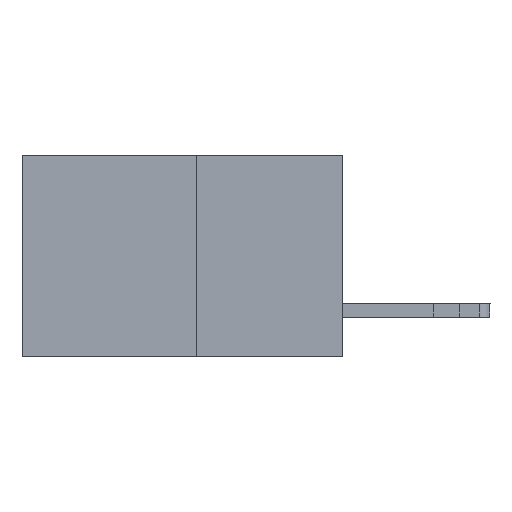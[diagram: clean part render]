
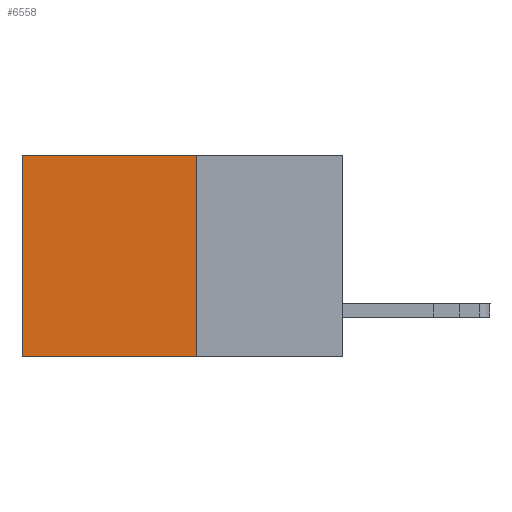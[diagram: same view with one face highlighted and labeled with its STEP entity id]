
A CAD part, left-side view. The second image highlights one B-rep face of the part: STEP entity #6558.
In plain terms, the highlighted planar face has unit normal (-1, 0, 0).
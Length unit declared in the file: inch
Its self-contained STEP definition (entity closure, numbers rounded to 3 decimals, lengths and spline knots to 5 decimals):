
#138 = EDGE_CURVE ( 'NONE', #12867, #1816, #12862, .T. ) ;
#195 = CARTESIAN_POINT ( 'NONE',  ( 0.277, 0.27, -0.37 ) ) ;
#1136 = PLANE ( 'NONE',  #14935 ) ;
#1172 = CARTESIAN_POINT ( 'NONE',  ( 0.277, 0.59, -0.37 ) ) ;
#1414 = DIRECTION ( 'NONE',  ( 0., 1., 0. ) ) ;
#1816 = VERTEX_POINT ( 'NONE', #1172 ) ;
#2304 = DIRECTION ( 'NONE',  ( 1., 0., 0. ) ) ;
#2605 = CARTESIAN_POINT ( 'NONE',  ( 0.277, 0.27, -0.37 ) ) ;
#2634 = LINE ( 'NONE', #12971, #4307 ) ;
#2694 = VERTEX_POINT ( 'NONE', #7727 ) ;
#2800 = FACE_OUTER_BOUND ( 'NONE', #6007, .T. ) ;
#4307 = VECTOR ( 'NONE', #8402, 39.37008 ) ;
#4363 = CARTESIAN_POINT ( 'NONE',  ( 0.277, 0.27, -0.37 ) ) ;
#5392 = EDGE_CURVE ( 'NONE', #11971, #1816, #10023, .T. ) ;
#5710 = EDGE_CURVE ( 'NONE', #2694, #11971, #11448, .T. ) ;
#6007 = EDGE_LOOP ( 'NONE', ( #6930, #14897, #6820, #9179 ) ) ;
#6021 = EDGE_CURVE ( 'NONE', #2694, #12867, #2634, .T. ) ;
#6418 = CARTESIAN_POINT ( 'NONE',  ( 0.277, 0.59, -0.37 ) ) ;
#6558 = ADVANCED_FACE ( 'NONE', ( #2800 ), #1136, .F. ) ;
#6820 = ORIENTED_EDGE ( 'NONE', *, *, #5710, .F. ) ;
#6930 = ORIENTED_EDGE ( 'NONE', *, *, #138, .T. ) ;
#7343 = DIRECTION ( 'NONE',  ( 0., 0., -1. ) ) ;
#7727 = CARTESIAN_POINT ( 'NONE',  ( 0.277, 0.27, 0. ) ) ;
#8227 = CARTESIAN_POINT ( 'NONE',  ( 0.277, 0.27, -0.37 ) ) ;
#8402 = DIRECTION ( 'NONE',  ( 0., 1., 0. ) ) ;
#9179 = ORIENTED_EDGE ( 'NONE', *, *, #6021, .T. ) ;
#10023 = LINE ( 'NONE', #2605, #12677 ) ;
#10541 = DIRECTION ( 'NONE',  ( 0., 0., -1. ) ) ;
#11134 = CARTESIAN_POINT ( 'NONE',  ( 0.277, 0.59, 0. ) ) ;
#11448 = LINE ( 'NONE', #4363, #14799 ) ;
#11971 = VERTEX_POINT ( 'NONE', #195 ) ;
#12476 = DIRECTION ( 'NONE',  ( 0., 0., -1. ) ) ;
#12497 = VECTOR ( 'NONE', #7343, 39.37008 ) ;
#12677 = VECTOR ( 'NONE', #1414, 39.37008 ) ;
#12862 = LINE ( 'NONE', #6418, #12497 ) ;
#12867 = VERTEX_POINT ( 'NONE', #11134 ) ;
#12971 = CARTESIAN_POINT ( 'NONE',  ( 0.277, 0.27, 0. ) ) ;
#14799 = VECTOR ( 'NONE', #12476, 39.37008 ) ;
#14897 = ORIENTED_EDGE ( 'NONE', *, *, #5392, .F. ) ;
#14935 = AXIS2_PLACEMENT_3D ( 'NONE', #8227, #2304, #10541 ) ;
